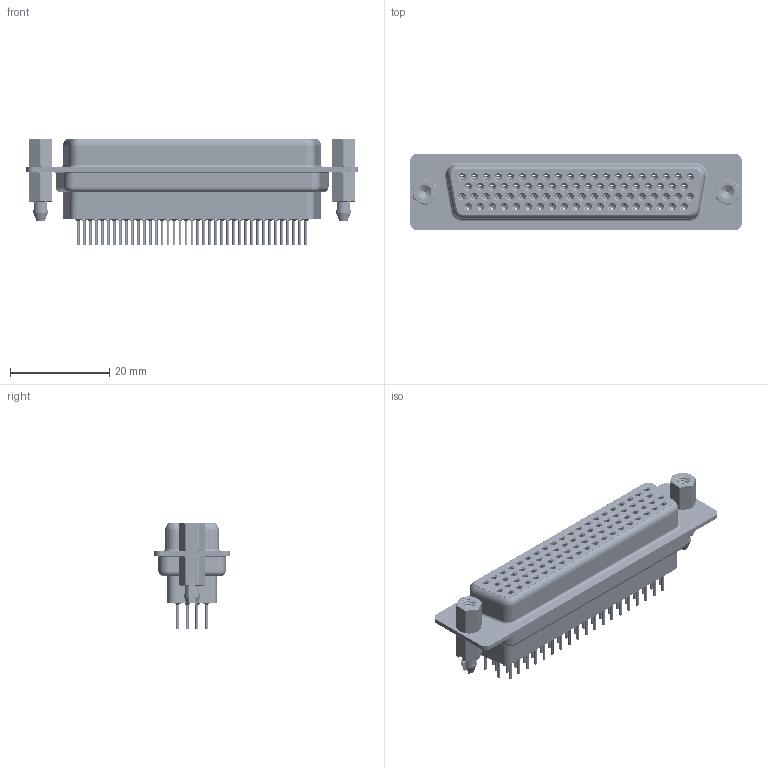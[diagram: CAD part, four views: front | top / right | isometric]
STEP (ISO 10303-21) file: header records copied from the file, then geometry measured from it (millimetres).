
FILE_DESCRIPTION (( 'STEP AP203' ), '1' );
FILE_NAME ('638-078-331-057.STEP', '2020-07-20T03:15:14', ( '' ), ( '' ), 'SwSTEP 2.0', 'SolidWorks 2020', '' );
FILE_SCHEMA (( 'CONFIG_CONTROL_DESIGN' ));
Length unit declared in the file: millimetre
Products named in the file (10): 638 4-40 Threaded Boardlock_LP; 638 Contact Row 2_31; 638-078-331-057; 638 Contact Row 78_31; 638 Shell Front_78 Contacts; 638 Housing_78 Contacts HP; 638 Contact Row 1_31; 638 Shell Rear_78 Contacts; 638 Contact Row 3_31; 638 4-40 Hex Standoff
Assembly tree (85 placements, depth 2):
  638-078-331-057
    638 Housing_78 Contacts HP
    638 Shell Front_78 Contacts
    638 Shell Rear_78 Contacts
    638 Contact Row 1_31  x19
    638 Contact Row 2_31  x20
    638 Contact Row 3_31  x19
    638 Contact Row 78_31  x20
    638 4-40 Hex Standoff  x2
    638 4-40 Threaded Boardlock_LP  x2
Bounding box: 67 x 15.4 x 21.5 mm (x, y, z)
Volume: 7635 mm3; surface area: 25781.5 mm2
Topology: 85 solids, 85 shells, 10073 faces, 25913 edges, 16175 vertices
Faces by surface type: cylinder 2815, plane 2539, torus 1929, bspline 1578, cone 1212
Entity records: 63383 total; most frequent: CARTESIAN_POINT 17977, DIRECTION 9374, ORIENTED_EDGE 8448, EDGE_CURVE 4224, AXIS2_PLACEMENT_3D 3950, VERTEX_POINT 2686, EDGE_LOOP 2214, CIRCLE 2151
